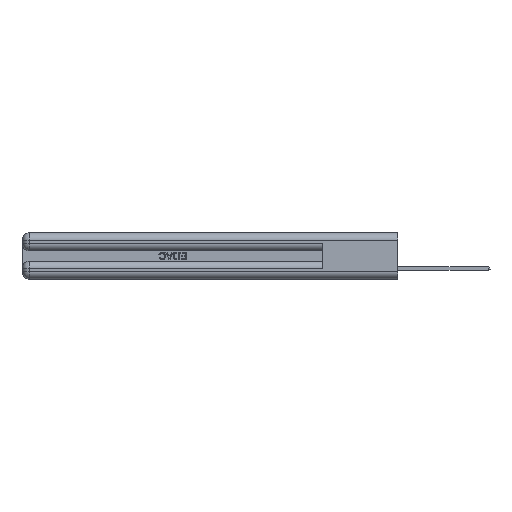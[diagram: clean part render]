
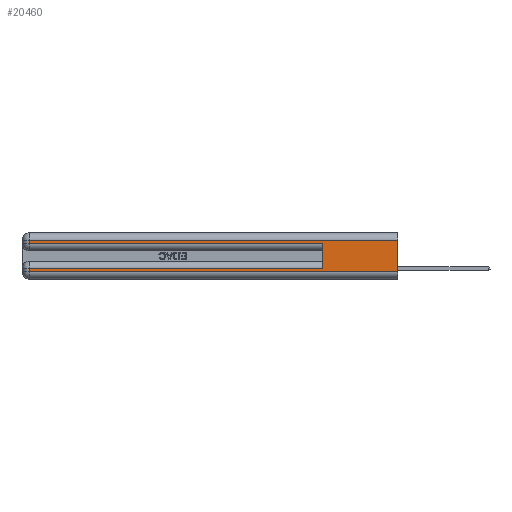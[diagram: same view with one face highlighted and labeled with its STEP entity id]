
A CAD part, left-side view. The second image highlights one B-rep face of the part: STEP entity #20460.
In plain terms, the highlighted planar face has unit normal (-1, 0, 0).
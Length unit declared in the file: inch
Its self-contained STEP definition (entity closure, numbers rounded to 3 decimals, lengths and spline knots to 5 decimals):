
#48 = CARTESIAN_POINT ( 'NONE',  ( 0., 0., 0.085 ) ) ;
#1066 = EDGE_CURVE ( 'NONE', #19712, #3999, #31721, .T. ) ;
#1142 = VERTEX_POINT ( 'NONE', #12963 ) ;
#1538 = VECTOR ( 'NONE', #28988, 39.37008 ) ;
#1653 = CARTESIAN_POINT ( 'NONE',  ( 0., 2.94, 0.31 ) ) ;
#2603 = EDGE_CURVE ( 'NONE', #40908, #28237, #25546, .T. ) ;
#2783 = DIRECTION ( 'NONE',  ( 0., -1., 0. ) ) ;
#3224 = VECTOR ( 'NONE', #2783, 39.37008 ) ;
#3393 = VECTOR ( 'NONE', #37126, 39.37008 ) ;
#3480 = ORIENTED_EDGE ( 'NONE', *, *, #4290, .T. ) ;
#3999 = VERTEX_POINT ( 'NONE', #26748 ) ;
#4101 = EDGE_CURVE ( 'NONE', #1142, #3999, #43292, .T. ) ;
#4290 = EDGE_CURVE ( 'NONE', #31301, #28237, #17297, .T. ) ;
#4395 = CARTESIAN_POINT ( 'NONE',  ( 0., 2.94, 0.085 ) ) ;
#5725 = ORIENTED_EDGE ( 'NONE', *, *, #10235, .T. ) ;
#6304 = CARTESIAN_POINT ( 'NONE',  ( 0., 2.94, 0.06 ) ) ;
#7561 = LINE ( 'NONE', #31983, #34101 ) ;
#9964 = EDGE_CURVE ( 'NONE', #40908, #41071, #20425, .T. ) ;
#10235 = EDGE_CURVE ( 'NONE', #1142, #25046, #25829, .T. ) ;
#12085 = ORIENTED_EDGE ( 'NONE', *, *, #4101, .F. ) ;
#12963 = CARTESIAN_POINT ( 'NONE',  ( 0., 0.6, 0.085 ) ) ;
#13107 = CARTESIAN_POINT ( 'NONE',  ( 0., 0., 0.31 ) ) ;
#13515 = AXIS2_PLACEMENT_3D ( 'NONE', #41067, #23295, #37275 ) ;
#14288 = DIRECTION ( 'NONE',  ( 0., 0., 1. ) ) ;
#15871 = CARTESIAN_POINT ( 'NONE',  ( 0., 0., 0.31 ) ) ;
#16688 = PLANE ( 'NONE',  #13515 ) ;
#16788 = EDGE_CURVE ( 'NONE', #25046, #31301, #7561, .T. ) ;
#17297 = LINE ( 'NONE', #30816, #3224 ) ;
#19712 = VERTEX_POINT ( 'NONE', #33975 ) ;
#20425 = LINE ( 'NONE', #15871, #1538 ) ;
#20460 = ADVANCED_FACE ( 'NONE', ( #44039 ), #16688, .F. ) ;
#20480 = DIRECTION ( 'NONE',  ( 0., -1., 0. ) ) ;
#21133 = ORIENTED_EDGE ( 'NONE', *, *, #16788, .T. ) ;
#21587 = DIRECTION ( 'NONE',  ( 0., 0., -1. ) ) ;
#21599 = VECTOR ( 'NONE', #14288, 39.37008 ) ;
#23295 = DIRECTION ( 'NONE',  ( 1., 0., 0. ) ) ;
#24081 = DIRECTION ( 'NONE',  ( 0., 1., 0. ) ) ;
#25046 = VERTEX_POINT ( 'NONE', #4395 ) ;
#25232 = ORIENTED_EDGE ( 'NONE', *, *, #1066, .T. ) ;
#25546 = LINE ( 'NONE', #33663, #3393 ) ;
#25829 = LINE ( 'NONE', #48, #26408 ) ;
#26408 = VECTOR ( 'NONE', #24081, 39.37008 ) ;
#26499 = VECTOR ( 'NONE', #31471, 39.37008 ) ;
#26748 = CARTESIAN_POINT ( 'NONE',  ( 0., 0.6, 0.285 ) ) ;
#27497 = CARTESIAN_POINT ( 'NONE',  ( 0., 0., 0.285 ) ) ;
#28237 = VERTEX_POINT ( 'NONE', #33563 ) ;
#28988 = DIRECTION ( 'NONE',  ( 0., 1., 0. ) ) ;
#30816 = CARTESIAN_POINT ( 'NONE',  ( 0., 0., 0.06 ) ) ;
#31301 = VERTEX_POINT ( 'NONE', #6304 ) ;
#31471 = DIRECTION ( 'NONE',  ( 0., 0., -1. ) ) ;
#31721 = LINE ( 'NONE', #27497, #39785 ) ;
#31983 = CARTESIAN_POINT ( 'NONE',  ( 0., 2.94, 0.37 ) ) ;
#33563 = CARTESIAN_POINT ( 'NONE',  ( 0., 0., 0.06 ) ) ;
#33663 = CARTESIAN_POINT ( 'NONE',  ( 0., 0., 0.37 ) ) ;
#33975 = CARTESIAN_POINT ( 'NONE',  ( 0., 2.94, 0.285 ) ) ;
#34101 = VECTOR ( 'NONE', #21587, 39.37008 ) ;
#34502 = CARTESIAN_POINT ( 'NONE',  ( 0., 2.94, 0.37 ) ) ;
#35859 = ORIENTED_EDGE ( 'NONE', *, *, #9964, .T. ) ;
#36322 = LINE ( 'NONE', #34502, #26499 ) ;
#36541 = ORIENTED_EDGE ( 'NONE', *, *, #37665, .T. ) ;
#37126 = DIRECTION ( 'NONE',  ( 0., 0., -1. ) ) ;
#37275 = DIRECTION ( 'NONE',  ( 0., 0., -1. ) ) ;
#37665 = EDGE_CURVE ( 'NONE', #41071, #19712, #36322, .T. ) ;
#39785 = VECTOR ( 'NONE', #20480, 39.37008 ) ;
#40029 = EDGE_LOOP ( 'NONE', ( #42369, #35859, #36541, #25232, #12085, #5725, #21133, #3480 ) ) ;
#40908 = VERTEX_POINT ( 'NONE', #13107 ) ;
#41067 = CARTESIAN_POINT ( 'NONE',  ( 0., 0., 0.37 ) ) ;
#41071 = VERTEX_POINT ( 'NONE', #1653 ) ;
#42369 = ORIENTED_EDGE ( 'NONE', *, *, #2603, .F. ) ;
#43292 = LINE ( 'NONE', #44835, #21599 ) ;
#44039 = FACE_OUTER_BOUND ( 'NONE', #40029, .T. ) ;
#44835 = CARTESIAN_POINT ( 'NONE',  ( 0., 0.6, 0.145 ) ) ;
